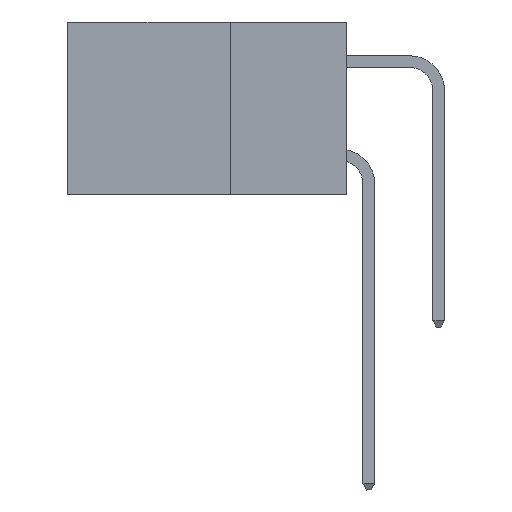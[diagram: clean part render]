
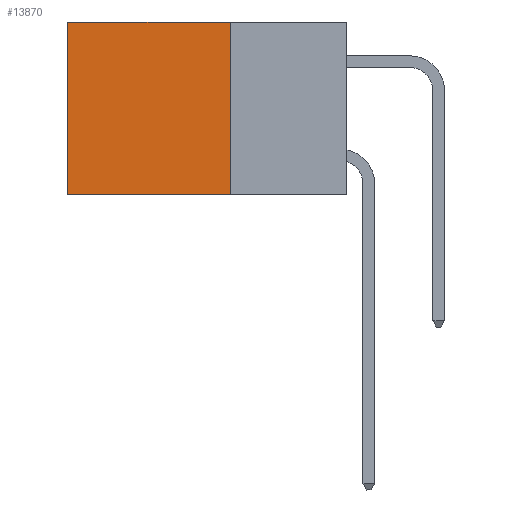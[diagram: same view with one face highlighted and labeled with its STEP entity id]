
A CAD part, left-side view. The second image highlights one B-rep face of the part: STEP entity #13870.
In plain terms, the highlighted planar face has unit normal (-1, 0, 0).
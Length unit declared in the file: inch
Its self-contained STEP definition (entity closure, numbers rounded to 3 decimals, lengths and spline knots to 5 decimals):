
#59 = DIRECTION ( 'NONE',  ( 0., 0., -1. ) ) ;
#632 = CARTESIAN_POINT ( 'NONE',  ( 0.2875, 0.6, 0. ) ) ;
#1405 = LINE ( 'NONE', #13702, #7374 ) ;
#1429 = VECTOR ( 'NONE', #10202, 39.37008 ) ;
#1872 = FACE_OUTER_BOUND ( 'NONE', #11810, .T. ) ;
#2642 = EDGE_CURVE ( 'NONE', #9232, #8110, #1405, .T. ) ;
#2650 = ORIENTED_EDGE ( 'NONE', *, *, #12991, .T. ) ;
#2717 = CARTESIAN_POINT ( 'NONE',  ( 0.2875, 0.25, -0.37 ) ) ;
#2745 = EDGE_CURVE ( 'NONE', #11200, #12755, #16429, .T. ) ;
#2816 = ORIENTED_EDGE ( 'NONE', *, *, #2745, .T. ) ;
#3119 = ORIENTED_EDGE ( 'NONE', *, *, #7807, .F. ) ;
#3462 = CARTESIAN_POINT ( 'NONE',  ( 0.2875, 0.25, -0.37 ) ) ;
#4941 = CARTESIAN_POINT ( 'NONE',  ( 0.2875, 0.25, 0. ) ) ;
#5113 = LINE ( 'NONE', #6908, #12929 ) ;
#5264 = DIRECTION ( 'NONE',  ( 0., 0., -1. ) ) ;
#6326 = DIRECTION ( 'NONE',  ( 0., 0., -1. ) ) ;
#6908 = CARTESIAN_POINT ( 'NONE',  ( 0.2875, 0.25, 0. ) ) ;
#7374 = VECTOR ( 'NONE', #59, 39.37008 ) ;
#7807 = EDGE_CURVE ( 'NONE', #8110, #12755, #8686, .T. ) ;
#8110 = VERTEX_POINT ( 'NONE', #2717 ) ;
#8686 = LINE ( 'NONE', #3462, #1429 ) ;
#9232 = VERTEX_POINT ( 'NONE', #12800 ) ;
#9817 = CARTESIAN_POINT ( 'NONE',  ( 0.2875, 0.6, 0. ) ) ;
#10202 = DIRECTION ( 'NONE',  ( 0., 1., 0. ) ) ;
#10303 = PLANE ( 'NONE',  #13079 ) ;
#11200 = VERTEX_POINT ( 'NONE', #632 ) ;
#11810 = EDGE_LOOP ( 'NONE', ( #2816, #3119, #16554, #2650 ) ) ;
#12755 = VERTEX_POINT ( 'NONE', #14065 ) ;
#12800 = CARTESIAN_POINT ( 'NONE',  ( 0.2875, 0.25, 0. ) ) ;
#12929 = VECTOR ( 'NONE', #15918, 39.37008 ) ;
#12991 = EDGE_CURVE ( 'NONE', #9232, #11200, #5113, .T. ) ;
#13041 = VECTOR ( 'NONE', #5264, 39.37008 ) ;
#13079 = AXIS2_PLACEMENT_3D ( 'NONE', #4941, #14117, #6326 ) ;
#13702 = CARTESIAN_POINT ( 'NONE',  ( 0.2875, 0.25, 0. ) ) ;
#13870 = ADVANCED_FACE ( 'NONE', ( #1872 ), #10303, .F. ) ;
#14065 = CARTESIAN_POINT ( 'NONE',  ( 0.2875, 0.6, -0.37 ) ) ;
#14117 = DIRECTION ( 'NONE',  ( 1., 0., 0. ) ) ;
#15918 = DIRECTION ( 'NONE',  ( 0., 1., 0. ) ) ;
#16429 = LINE ( 'NONE', #9817, #13041 ) ;
#16554 = ORIENTED_EDGE ( 'NONE', *, *, #2642, .F. ) ;
